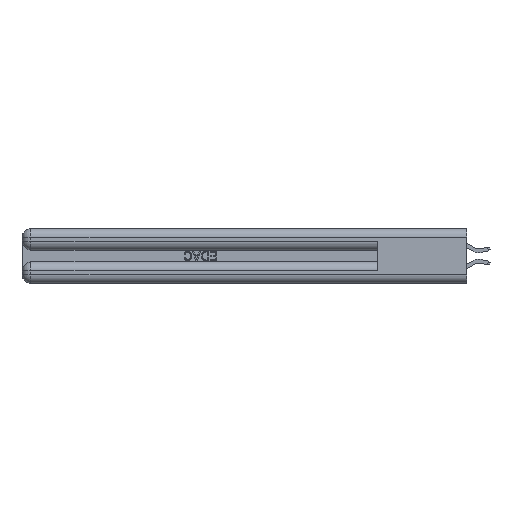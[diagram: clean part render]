
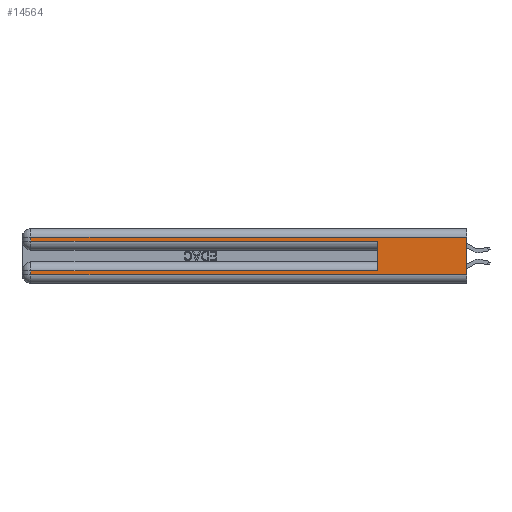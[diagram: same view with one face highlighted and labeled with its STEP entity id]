
A CAD part, left-side view. The second image highlights one B-rep face of the part: STEP entity #14564.
In plain terms, the highlighted planar face has unit normal (-1, 0, 0).
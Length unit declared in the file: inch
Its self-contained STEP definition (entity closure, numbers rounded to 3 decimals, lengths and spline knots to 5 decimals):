
#267 = VERTEX_POINT ( 'NONE', #28473 ) ;
#828 = VECTOR ( 'NONE', #4234, 39.37008 ) ;
#1392 = CARTESIAN_POINT ( 'NONE',  ( 0., 0., 0.06 ) ) ;
#1966 = CARTESIAN_POINT ( 'NONE',  ( 0., 0., 0.31 ) ) ;
#2189 = VERTEX_POINT ( 'NONE', #23598 ) ;
#4013 = AXIS2_PLACEMENT_3D ( 'NONE', #12978, #37043, #16562 ) ;
#4234 = DIRECTION ( 'NONE',  ( 0., 0., 1. ) ) ;
#4888 = EDGE_CURVE ( 'NONE', #2189, #28749, #19526, .T. ) ;
#6475 = VERTEX_POINT ( 'NONE', #9997 ) ;
#6880 = VERTEX_POINT ( 'NONE', #40734 ) ;
#8683 = LINE ( 'NONE', #1966, #15609 ) ;
#8755 = DIRECTION ( 'NONE',  ( 0., 0., -1. ) ) ;
#8938 = CARTESIAN_POINT ( 'NONE',  ( 0., 0., 0.085 ) ) ;
#9997 = CARTESIAN_POINT ( 'NONE',  ( 0., 2.94, 0.31 ) ) ;
#10773 = VERTEX_POINT ( 'NONE', #24142 ) ;
#11090 = VECTOR ( 'NONE', #33651, 39.37008 ) ;
#11497 = ORIENTED_EDGE ( 'NONE', *, *, #42616, .T. ) ;
#11644 = LINE ( 'NONE', #12192, #28764 ) ;
#11693 = CARTESIAN_POINT ( 'NONE',  ( 0., 0., 0.06 ) ) ;
#12192 = CARTESIAN_POINT ( 'NONE',  ( 0., 2.94, 0.37 ) ) ;
#12275 = DIRECTION ( 'NONE',  ( 0., 1., 0. ) ) ;
#12978 = CARTESIAN_POINT ( 'NONE',  ( 0., 0., 0.37 ) ) ;
#13118 = PLANE ( 'NONE',  #4013 ) ;
#14564 = ADVANCED_FACE ( 'NONE', ( #19669 ), #13118, .F. ) ;
#15108 = DIRECTION ( 'NONE',  ( 0., -1., 0. ) ) ;
#15609 = VECTOR ( 'NONE', #12275, 39.37008 ) ;
#16409 = VECTOR ( 'NONE', #19241, 39.37008 ) ;
#16562 = DIRECTION ( 'NONE',  ( 0., 0., -1. ) ) ;
#16760 = ORIENTED_EDGE ( 'NONE', *, *, #16946, .T. ) ;
#16946 = EDGE_CURVE ( 'NONE', #37385, #32016, #40339, .T. ) ;
#17101 = CARTESIAN_POINT ( 'NONE',  ( 0., 2.94, 0.285 ) ) ;
#17485 = LINE ( 'NONE', #8938, #16409 ) ;
#19241 = DIRECTION ( 'NONE',  ( 0., 1., 0. ) ) ;
#19375 = EDGE_CURVE ( 'NONE', #10773, #6880, #27129, .T. ) ;
#19526 = LINE ( 'NONE', #29246, #20600 ) ;
#19669 = FACE_OUTER_BOUND ( 'NONE', #33581, .T. ) ;
#19912 = EDGE_CURVE ( 'NONE', #267, #10773, #17485, .T. ) ;
#20600 = VECTOR ( 'NONE', #8755, 39.37008 ) ;
#21260 = CARTESIAN_POINT ( 'NONE',  ( 0., 0.6, 0.145 ) ) ;
#23191 = ORIENTED_EDGE ( 'NONE', *, *, #19912, .T. ) ;
#23598 = CARTESIAN_POINT ( 'NONE',  ( 0., 0., 0.31 ) ) ;
#24142 = CARTESIAN_POINT ( 'NONE',  ( 0., 2.94, 0.085 ) ) ;
#24724 = VECTOR ( 'NONE', #15108, 39.37008 ) ;
#26633 = CARTESIAN_POINT ( 'NONE',  ( 0., 0., 0.285 ) ) ;
#26776 = DIRECTION ( 'NONE',  ( 0., -1., 0. ) ) ;
#27129 = LINE ( 'NONE', #30229, #11090 ) ;
#28473 = CARTESIAN_POINT ( 'NONE',  ( 0., 0.6, 0.085 ) ) ;
#28749 = VERTEX_POINT ( 'NONE', #1392 ) ;
#28764 = VECTOR ( 'NONE', #29248, 39.37008 ) ;
#29246 = CARTESIAN_POINT ( 'NONE',  ( 0., 0., 0.37 ) ) ;
#29248 = DIRECTION ( 'NONE',  ( 0., 0., -1. ) ) ;
#29619 = ORIENTED_EDGE ( 'NONE', *, *, #35935, .F. ) ;
#30229 = CARTESIAN_POINT ( 'NONE',  ( 0., 2.94, 0.37 ) ) ;
#31282 = ORIENTED_EDGE ( 'NONE', *, *, #4888, .F. ) ;
#31295 = VECTOR ( 'NONE', #26776, 39.37008 ) ;
#31445 = EDGE_CURVE ( 'NONE', #6880, #28749, #42881, .T. ) ;
#32016 = VERTEX_POINT ( 'NONE', #34930 ) ;
#33581 = EDGE_LOOP ( 'NONE', ( #31282, #11497, #44103, #16760, #29619, #23191, #43496, #42999 ) ) ;
#33651 = DIRECTION ( 'NONE',  ( 0., 0., -1. ) ) ;
#34930 = CARTESIAN_POINT ( 'NONE',  ( 0., 0.6, 0.285 ) ) ;
#35935 = EDGE_CURVE ( 'NONE', #267, #32016, #37185, .T. ) ;
#37043 = DIRECTION ( 'NONE',  ( 1., 0., 0. ) ) ;
#37185 = LINE ( 'NONE', #21260, #828 ) ;
#37385 = VERTEX_POINT ( 'NONE', #17101 ) ;
#39603 = EDGE_CURVE ( 'NONE', #6475, #37385, #11644, .T. ) ;
#40339 = LINE ( 'NONE', #26633, #31295 ) ;
#40734 = CARTESIAN_POINT ( 'NONE',  ( 0., 2.94, 0.06 ) ) ;
#42616 = EDGE_CURVE ( 'NONE', #2189, #6475, #8683, .T. ) ;
#42881 = LINE ( 'NONE', #11693, #24724 ) ;
#42999 = ORIENTED_EDGE ( 'NONE', *, *, #31445, .T. ) ;
#43496 = ORIENTED_EDGE ( 'NONE', *, *, #19375, .T. ) ;
#44103 = ORIENTED_EDGE ( 'NONE', *, *, #39603, .T. ) ;
